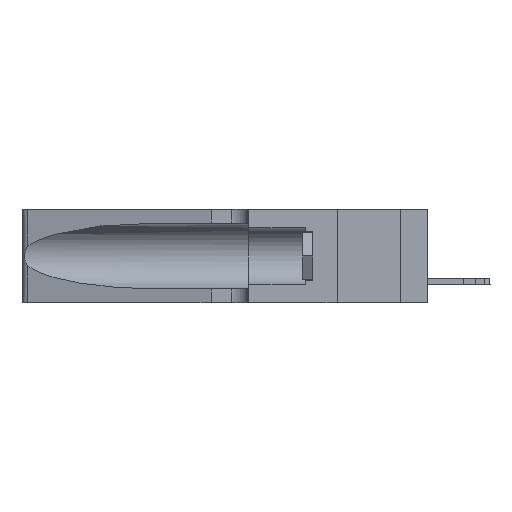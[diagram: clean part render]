
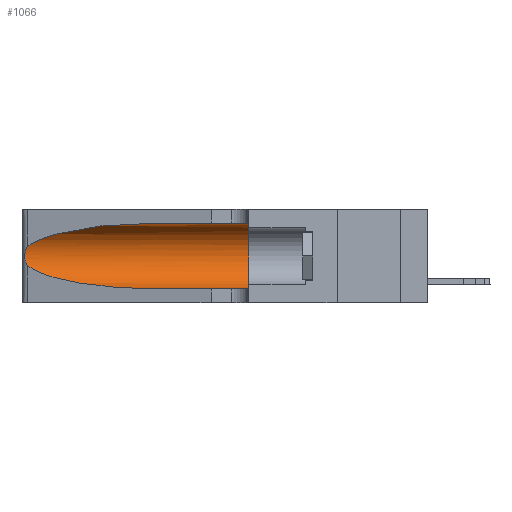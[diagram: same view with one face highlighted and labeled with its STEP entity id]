
A CAD part, left-side view. The second image highlights one B-rep face of the part: STEP entity #1066.
In plain terms, the highlighted cylindrical face has radius 3.308 mm (diameter 6.617 mm), a partial arc.
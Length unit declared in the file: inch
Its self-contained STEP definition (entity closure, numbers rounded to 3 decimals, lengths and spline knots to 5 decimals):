
#31 = EDGE_CURVE ( 'NONE', #7115, #12014, #3904, .T. ) ;
#698 = AXIS2_PLACEMENT_3D ( 'NONE', #34358, #15579, #37501 ) ;
#1066 = ADVANCED_FACE ( 'NONE', ( #2322 ), #38616, .F. ) ;
#1758 = VERTEX_POINT ( 'NONE', #7587 ) ;
#2004 = VERTEX_POINT ( 'NONE', #7398 ) ;
#2322 = FACE_OUTER_BOUND ( 'NONE', #24921, .T. ) ;
#3904 = CIRCLE ( 'NONE', #7512, 0.13025 ) ;
#4284 = CARTESIAN_POINT ( 'NONE',  ( 0.2373, 1.15595, 0.28018 ) ) ;
#5394 = B_SPLINE_CURVE_WITH_KNOTS ( 'NONE', 3,
 ( #33696, #40138, #24559, #40284, #27680, #17933, #18490, #40418, #14806, #30812, #21657, #18352, #40007, #24833 ),
 .UNSPECIFIED., .F., .F.,
 ( 4, 2, 2, 2, 2, 2, 4 ),
 ( 0., 0.00027, 0.00053, 0.00107, 0.0016, 0.00187, 0.00214 ),
 .UNSPECIFIED. ) ;
#7115 = VERTEX_POINT ( 'NONE', #38383 ) ;
#7398 = CARTESIAN_POINT ( 'NONE',  ( 0.1305, 0.72297, 0.05475 ) ) ;
#7512 = AXIS2_PLACEMENT_3D ( 'NONE', #27647, #12180, #30783 ) ;
#7587 = CARTESIAN_POINT ( 'NONE',  ( 0.25487, 1.22718, 0.14631 ) ) ;
#8326 = CARTESIAN_POINT ( 'NONE',  ( 0.18966, 0.96281, 0.05475 ) ) ;
#8611 = EDGE_CURVE ( 'NONE', #13039, #7115, #33039, .T. ) ;
#10956 = CARTESIAN_POINT ( 'NONE',  ( 0.1305, 0.72297, 0.31525 ) ) ;
#11306 = CARTESIAN_POINT ( 'NONE',  ( 0.2373, 1.15595, 0.08982 ) ) ;
#12014 = VERTEX_POINT ( 'NONE', #20489 ) ;
#12180 = DIRECTION ( 'NONE',  ( 0., 1., 0. ) ) ;
#12764 = ORIENTED_EDGE ( 'NONE', *, *, #31, .F. ) ;
#13039 = VERTEX_POINT ( 'NONE', #10956 ) ;
#13248 = ORIENTED_EDGE ( 'NONE', *, *, #8611, .F. ) ;
#14324 = CARTESIAN_POINT ( 'NONE',  ( 0.25487, 1.22718, 0.14631 ) ) ;
#14806 = CARTESIAN_POINT ( 'NONE',  ( 0.26017, 1.23833, 0.17102 ) ) ;
#14852 = EDGE_CURVE ( 'NONE', #1758, #2004, #32497, .T. ) ;
#15579 = DIRECTION ( 'NONE',  ( 0., -1., 0. ) ) ;
#16464 = CARTESIAN_POINT ( 'NONE',  ( 0.25487, 1.22718, 0.22369 ) ) ;
#16743 = CARTESIAN_POINT ( 'NONE',  ( 0.1305, 1.61858, 0.31525 ) ) ;
#16885 = DIRECTION ( 'NONE',  ( 0., -1., 0. ) ) ;
#17933 = CARTESIAN_POINT ( 'NONE',  ( 0.26018, 1.23835, 0.19895 ) ) ;
#18352 = CARTESIAN_POINT ( 'NONE',  ( 0.25639, 1.23186, 0.15144 ) ) ;
#18490 = CARTESIAN_POINT ( 'NONE',  ( 0.26075, 1.23896, 0.19203 ) ) ;
#18698 = EDGE_CURVE ( 'NONE', #13039, #32479, #22976, .T. ) ;
#19402 = CARTESIAN_POINT ( 'NONE',  ( 0.25487, 1.22718, 0.22369 ) ) ;
#19795 = CARTESIAN_POINT ( 'NONE',  ( 0.1305, 0.72297, 0.31525 ) ) ;
#20489 = CARTESIAN_POINT ( 'NONE',  ( 0.1305, 0.35, 0.05475 ) ) ;
#20668 = CARTESIAN_POINT ( 'NONE',  ( 0.1305, 1.61858, 0.05475 ) ) ;
#21657 = CARTESIAN_POINT ( 'NONE',  ( 0.25789, 1.23486, 0.15765 ) ) ;
#22543 = ORIENTED_EDGE ( 'NONE', *, *, #31787, .T. ) ;
#22976 =( BOUNDED_CURVE ( )  B_SPLINE_CURVE ( 3, ( #19795, #23090, #4284, #16464 ),
 .UNSPECIFIED., .F., .F. ) 
 B_SPLINE_CURVE_WITH_KNOTS ( ( 4, 4 ),
 ( 1.5708, 2.84003 ),
 .UNSPECIFIED. ) 
 CURVE ( )  GEOMETRIC_REPRESENTATION_ITEM ( )  RATIONAL_B_SPLINE_CURVE ( ( 1., 0.87, 0.87, 1. ) ) 
 REPRESENTATION_ITEM ( '' )  );
#23090 = CARTESIAN_POINT ( 'NONE',  ( 0.18966, 0.96281, 0.31525 ) ) ;
#24559 = CARTESIAN_POINT ( 'NONE',  ( 0.25639, 1.23184, 0.21858 ) ) ;
#24833 = CARTESIAN_POINT ( 'NONE',  ( 0.25487, 1.22718, 0.14631 ) ) ;
#24921 = EDGE_LOOP ( 'NONE', ( #35104, #22543, #37788, #36073, #12764, #13248 ) ) ;
#27647 = CARTESIAN_POINT ( 'NONE',  ( 0.1305, 0.35, 0.185 ) ) ;
#27680 = CARTESIAN_POINT ( 'NONE',  ( 0.25854, 1.2359, 0.20912 ) ) ;
#29098 = VECTOR ( 'NONE', #16885, 39.37008 ) ;
#30265 = EDGE_CURVE ( 'NONE', #2004, #12014, #39584, .T. ) ;
#30783 = DIRECTION ( 'NONE',  ( 0., 0., 1. ) ) ;
#30812 = CARTESIAN_POINT ( 'NONE',  ( 0.25856, 1.23593, 0.16098 ) ) ;
#31787 = EDGE_CURVE ( 'NONE', #32479, #1758, #5394, .T. ) ;
#32218 = VECTOR ( 'NONE', #36534, 39.37008 ) ;
#32479 = VERTEX_POINT ( 'NONE', #19402 ) ;
#32497 =( BOUNDED_CURVE ( )  B_SPLINE_CURVE ( 3, ( #14324, #11306, #8326, #33628 ),
 .UNSPECIFIED., .F., .F. ) 
 B_SPLINE_CURVE_WITH_KNOTS ( ( 4, 4 ),
 ( 3.44316, 4.71239 ),
 .UNSPECIFIED. ) 
 CURVE ( )  GEOMETRIC_REPRESENTATION_ITEM ( )  RATIONAL_B_SPLINE_CURVE ( ( 1., 0.87, 0.87, 1. ) ) 
 REPRESENTATION_ITEM ( '' )  );
#33039 = LINE ( 'NONE', #16743, #29098 ) ;
#33628 = CARTESIAN_POINT ( 'NONE',  ( 0.1305, 0.72297, 0.05475 ) ) ;
#33696 = CARTESIAN_POINT ( 'NONE',  ( 0.25487, 1.22718, 0.22369 ) ) ;
#34358 = CARTESIAN_POINT ( 'NONE',  ( 0.1305, 1.61858, 0.185 ) ) ;
#35104 = ORIENTED_EDGE ( 'NONE', *, *, #18698, .T. ) ;
#36073 = ORIENTED_EDGE ( 'NONE', *, *, #30265, .T. ) ;
#36534 = DIRECTION ( 'NONE',  ( 0., -1., 0. ) ) ;
#37501 = DIRECTION ( 'NONE',  ( 0., 0., -1. ) ) ;
#37788 = ORIENTED_EDGE ( 'NONE', *, *, #14852, .T. ) ;
#38383 = CARTESIAN_POINT ( 'NONE',  ( 0.1305, 0.35, 0.31525 ) ) ;
#38616 = CYLINDRICAL_SURFACE ( 'NONE', #698, 0.13025 ) ;
#39584 = LINE ( 'NONE', #20668, #32218 ) ;
#40007 = CARTESIAN_POINT ( 'NONE',  ( 0.25555, 1.22993, 0.14849 ) ) ;
#40138 = CARTESIAN_POINT ( 'NONE',  ( 0.25555, 1.22994, 0.2215 ) ) ;
#40284 = CARTESIAN_POINT ( 'NONE',  ( 0.25787, 1.23484, 0.2124 ) ) ;
#40418 = CARTESIAN_POINT ( 'NONE',  ( 0.26075, 1.23896, 0.178 ) ) ;
